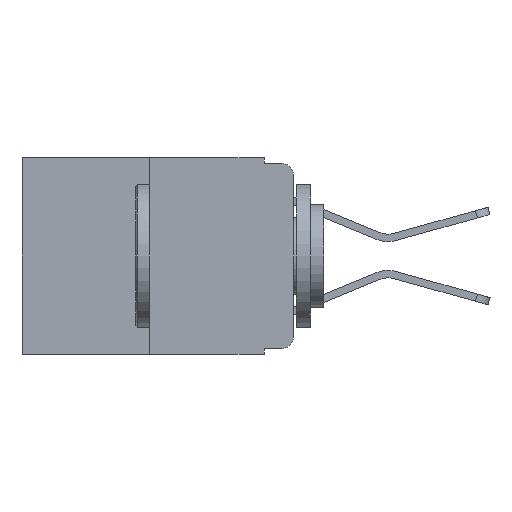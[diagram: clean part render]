
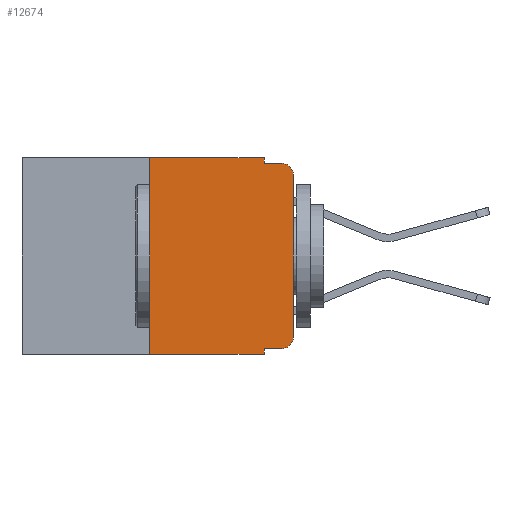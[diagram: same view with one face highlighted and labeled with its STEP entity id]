
A CAD part, left-side view. The second image highlights one B-rep face of the part: STEP entity #12674.
In plain terms, the highlighted planar face has unit normal (-1, 0, 0).
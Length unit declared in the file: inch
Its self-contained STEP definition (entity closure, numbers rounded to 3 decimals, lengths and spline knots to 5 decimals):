
#29 = DIRECTION ( 'NONE',  ( -1., 0., 0. ) ) ;
#41 = VECTOR ( 'NONE', #773, 39.37008 ) ;
#239 = LINE ( 'NONE', #12255, #6663 ) ;
#479 = CARTESIAN_POINT ( 'NONE',  ( 0., 0.051, 0. ) ) ;
#668 = VERTEX_POINT ( 'NONE', #8289 ) ;
#753 = CARTESIAN_POINT ( 'NONE',  ( 0., 0., -0.313 ) ) ;
#773 = DIRECTION ( 'NONE',  ( 0., 0., 1. ) ) ;
#776 = VECTOR ( 'NONE', #10308, 39.37008 ) ;
#1050 = ORIENTED_EDGE ( 'NONE', *, *, #8100, .T. ) ;
#1114 = LINE ( 'NONE', #479, #2171 ) ;
#1573 = ORIENTED_EDGE ( 'NONE', *, *, #12810, .T. ) ;
#1723 = ORIENTED_EDGE ( 'NONE', *, *, #2963, .F. ) ;
#1824 = EDGE_CURVE ( 'NONE', #14092, #8613, #1114, .T. ) ;
#2008 = VECTOR ( 'NONE', #9825, 39.37008 ) ;
#2121 = CARTESIAN_POINT ( 'NONE',  ( 0., 0.25, 0. ) ) ;
#2132 = ORIENTED_EDGE ( 'NONE', *, *, #2359, .F. ) ;
#2171 = VECTOR ( 'NONE', #5120, 39.37008 ) ;
#2224 = CARTESIAN_POINT ( 'NONE',  ( 0., 0.051, -0.01 ) ) ;
#2245 = ORIENTED_EDGE ( 'NONE', *, *, #9895, .T. ) ;
#2359 = EDGE_CURVE ( 'NONE', #5251, #12806, #13411, .T. ) ;
#2527 = AXIS2_PLACEMENT_3D ( 'NONE', #2564, #10872, #8662 ) ;
#2564 = CARTESIAN_POINT ( 'NONE',  ( 0., 0.02, -0.313 ) ) ;
#2902 = LINE ( 'NONE', #14733, #8436 ) ;
#2963 = EDGE_CURVE ( 'NONE', #12806, #4721, #5184, .T. ) ;
#4109 = CARTESIAN_POINT ( 'NONE',  ( 0., 0.473, 0. ) ) ;
#4125 = ORIENTED_EDGE ( 'NONE', *, *, #7968, .F. ) ;
#4247 = DIRECTION ( 'NONE',  ( 0., 0., -1. ) ) ;
#4251 = VERTEX_POINT ( 'NONE', #753 ) ;
#4402 = CARTESIAN_POINT ( 'NONE',  ( 0., 0.02, -0.03 ) ) ;
#4438 = ORIENTED_EDGE ( 'NONE', *, *, #1824, .F. ) ;
#4721 = VERTEX_POINT ( 'NONE', #7786 ) ;
#4952 = CARTESIAN_POINT ( 'NONE',  ( 0., 0.051, -0.333 ) ) ;
#5120 = DIRECTION ( 'NONE',  ( 0., 0., -1. ) ) ;
#5184 = LINE ( 'NONE', #4109, #5545 ) ;
#5251 = VERTEX_POINT ( 'NONE', #9807 ) ;
#5389 = VECTOR ( 'NONE', #8871, 39.37008 ) ;
#5487 = PLANE ( 'NONE',  #9289 ) ;
#5545 = VECTOR ( 'NONE', #14316, 39.37008 ) ;
#6663 = VECTOR ( 'NONE', #4247, 39.37008 ) ;
#7550 = CARTESIAN_POINT ( 'NONE',  ( 0., 0., 0. ) ) ;
#7786 = CARTESIAN_POINT ( 'NONE',  ( 0., 0.051, 0. ) ) ;
#7811 = ORIENTED_EDGE ( 'NONE', *, *, #7974, .T. ) ;
#7968 = EDGE_CURVE ( 'NONE', #4721, #12830, #239, .T. ) ;
#7974 = EDGE_CURVE ( 'NONE', #5251, #8613, #13991, .T. ) ;
#8072 = ORIENTED_EDGE ( 'NONE', *, *, #10143, .T. ) ;
#8100 = EDGE_CURVE ( 'NONE', #668, #11789, #9505, .T. ) ;
#8289 = CARTESIAN_POINT ( 'NONE',  ( 0., 0., -0.03 ) ) ;
#8436 = VECTOR ( 'NONE', #11284, 39.37008 ) ;
#8613 = VERTEX_POINT ( 'NONE', #14636 ) ;
#8662 = DIRECTION ( 'NONE',  ( 0., 0., -1. ) ) ;
#8871 = DIRECTION ( 'NONE',  ( 0., 0., 1. ) ) ;
#9020 = CARTESIAN_POINT ( 'NONE',  ( 0., 0.051, -0.01 ) ) ;
#9233 = CARTESIAN_POINT ( 'NONE',  ( 0., 0.02, -0.333 ) ) ;
#9289 = AXIS2_PLACEMENT_3D ( 'NONE', #13470, #12181, #11085 ) ;
#9479 = LINE ( 'NONE', #7550, #41 ) ;
#9505 = CIRCLE ( 'NONE', #12956, 0.02 ) ;
#9513 = FACE_OUTER_BOUND ( 'NONE', #13123, .T. ) ;
#9807 = CARTESIAN_POINT ( 'NONE',  ( 0., 0.25, -0.343 ) ) ;
#9810 = CIRCLE ( 'NONE', #2527, 0.02 ) ;
#9825 = DIRECTION ( 'NONE',  ( 0., -1., 0. ) ) ;
#9895 = EDGE_CURVE ( 'NONE', #4251, #668, #9479, .T. ) ;
#10143 = EDGE_CURVE ( 'NONE', #12226, #4251, #9810, .T. ) ;
#10308 = DIRECTION ( 'NONE',  ( 0., -1., 0. ) ) ;
#10872 = DIRECTION ( 'NONE',  ( -1., 0., 0. ) ) ;
#11085 = DIRECTION ( 'NONE',  ( 0., 0., -1. ) ) ;
#11284 = DIRECTION ( 'NONE',  ( 0., -1., 0. ) ) ;
#11789 = VERTEX_POINT ( 'NONE', #13094 ) ;
#11875 = ORIENTED_EDGE ( 'NONE', *, *, #12693, .F. ) ;
#12181 = DIRECTION ( 'NONE',  ( 1., 0., 0. ) ) ;
#12226 = VERTEX_POINT ( 'NONE', #9233 ) ;
#12255 = CARTESIAN_POINT ( 'NONE',  ( 0., 0.051, 0. ) ) ;
#12393 = LINE ( 'NONE', #9020, #776 ) ;
#12674 = ADVANCED_FACE ( 'NONE', ( #9513 ), #5487, .F. ) ;
#12693 = EDGE_CURVE ( 'NONE', #12830, #11789, #12393, .T. ) ;
#12806 = VERTEX_POINT ( 'NONE', #2121 ) ;
#12810 = EDGE_CURVE ( 'NONE', #14092, #12226, #2902, .T. ) ;
#12830 = VERTEX_POINT ( 'NONE', #2224 ) ;
#12956 = AXIS2_PLACEMENT_3D ( 'NONE', #4402, #29, #13545 ) ;
#13074 = CARTESIAN_POINT ( 'NONE',  ( 0., 0.25, 0. ) ) ;
#13094 = CARTESIAN_POINT ( 'NONE',  ( 0., 0.02, -0.01 ) ) ;
#13123 = EDGE_LOOP ( 'NONE', ( #2245, #1050, #11875, #4125, #1723, #2132, #7811, #4438, #1573, #8072 ) ) ;
#13296 = CARTESIAN_POINT ( 'NONE',  ( 0., 0.473, -0.343 ) ) ;
#13411 = LINE ( 'NONE', #13074, #5389 ) ;
#13470 = CARTESIAN_POINT ( 'NONE',  ( 0., 0.473, 0. ) ) ;
#13545 = DIRECTION ( 'NONE',  ( 0., 0., -1. ) ) ;
#13991 = LINE ( 'NONE', #13296, #2008 ) ;
#14092 = VERTEX_POINT ( 'NONE', #4952 ) ;
#14316 = DIRECTION ( 'NONE',  ( 0., -1., 0. ) ) ;
#14636 = CARTESIAN_POINT ( 'NONE',  ( 0., 0.051, -0.343 ) ) ;
#14733 = CARTESIAN_POINT ( 'NONE',  ( 0., 0.051, -0.333 ) ) ;
